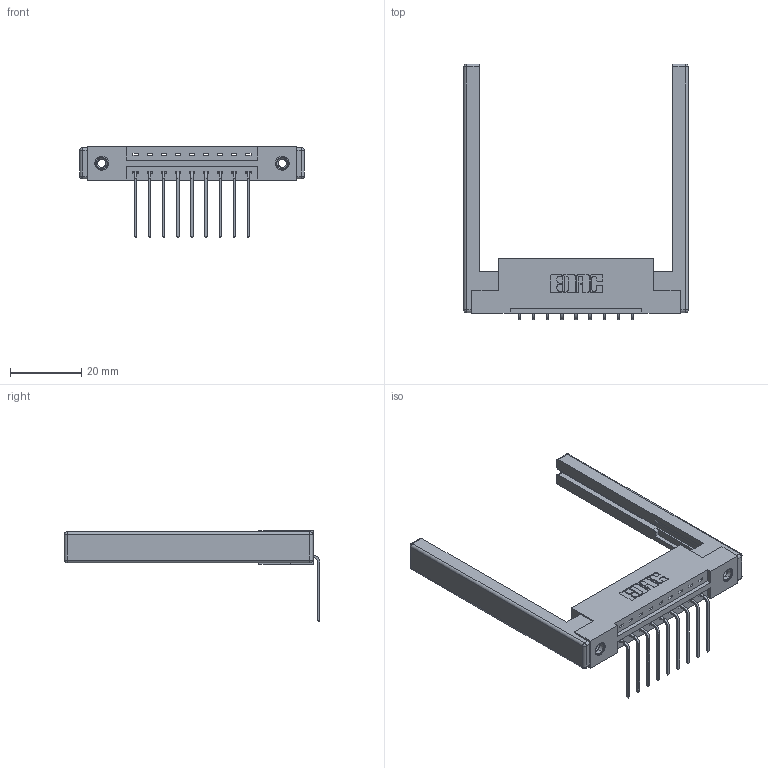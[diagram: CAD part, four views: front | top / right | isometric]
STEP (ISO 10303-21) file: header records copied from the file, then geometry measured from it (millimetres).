
FILE_DESCRIPTION (( 'STEP AP203' ), '1' );
FILE_NAME ('337-009-559-168.STEP', '2019-09-27T20:42:48', ( '' ), ( '' ), 'SwSTEP 2.0', 'SolidWorks 2016', '' );
FILE_SCHEMA (( 'CONFIG_CONTROL_DESIGN' ));
Length unit declared in the file: inch
Products named in the file (5): 337 Part_Flush Mounting Lugs - 0.156 Dia-TI; 307-220-068; 345-250-001_345-250-001-102; 345-292-001_558 559 Tail - 1; 337-009-559-168
Assembly tree (14 placements, depth 2):
  337-009-559-168
    337 Part_Flush Mounting Lugs - 0.156 Dia-TI
    345-292-001_558 559 Tail - 1  x9
    345-250-001_345-250-001-102  x2
    307-220-068  x2
Bounding box: 63.09 x 71.82 x 25.53 mm (x, y, z)
Volume: 10565.8 mm3; surface area: 10474.2 mm2
Topology: 14 solids, 14 shells, 844 faces, 2447 edges, 1598 vertices
Faces by surface type: plane 590, cylinder 230, cone 12, sphere 8, torus 4
Entity records: 13802 total; most frequent: CARTESIAN_POINT 2358, ORIENTED_EDGE 2292, DIRECTION 2126, EDGE_CURVE 1146, LINE 968, VECTOR 968, VERTEX_POINT 754, AXIS2_PLACEMENT_3D 579
